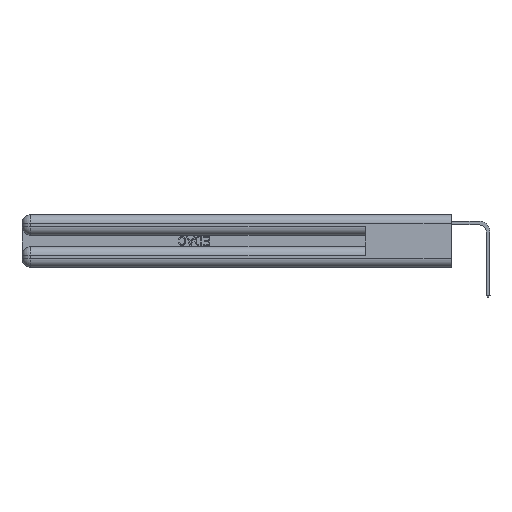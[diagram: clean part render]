
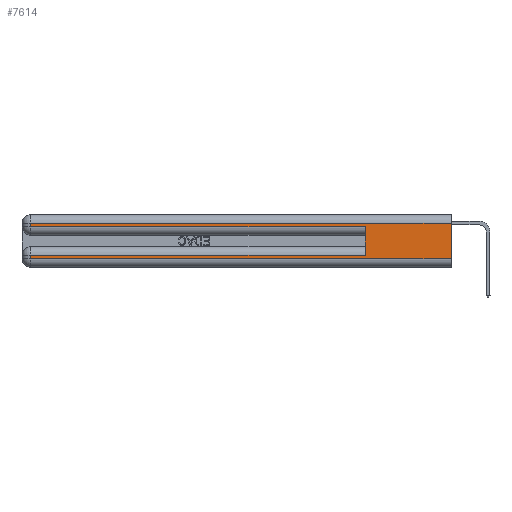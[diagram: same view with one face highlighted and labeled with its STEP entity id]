
A CAD part, left-side view. The second image highlights one B-rep face of the part: STEP entity #7614.
In plain terms, the highlighted planar face has unit normal (-1, 0, 0).
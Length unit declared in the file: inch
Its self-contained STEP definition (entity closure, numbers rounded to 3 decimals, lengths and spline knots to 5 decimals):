
#253 = CARTESIAN_POINT ( 'NONE',  ( 0., 2.94, 0.31 ) ) ;
#452 = VERTEX_POINT ( 'NONE', #21533 ) ;
#843 = EDGE_CURVE ( 'NONE', #30634, #452, #5601, .T. ) ;
#1030 = VERTEX_POINT ( 'NONE', #19496 ) ;
#1300 = EDGE_CURVE ( 'NONE', #452, #10364, #24338, .T. ) ;
#1355 = VECTOR ( 'NONE', #16055, 39.37008 ) ;
#1785 = VECTOR ( 'NONE', #31745, 39.37008 ) ;
#2226 = LINE ( 'NONE', #19199, #3964 ) ;
#2249 = CARTESIAN_POINT ( 'NONE',  ( 0., 0.6, 0.085 ) ) ;
#2489 = CARTESIAN_POINT ( 'NONE',  ( 0., 2.94, 0.37 ) ) ;
#3964 = VECTOR ( 'NONE', #19020, 39.37008 ) ;
#4305 = LINE ( 'NONE', #32068, #22374 ) ;
#4582 = EDGE_CURVE ( 'NONE', #30634, #18506, #25708, .T. ) ;
#4866 = CARTESIAN_POINT ( 'NONE',  ( 0., 2.94, 0.06 ) ) ;
#5601 = LINE ( 'NONE', #30299, #11284 ) ;
#5830 = VERTEX_POINT ( 'NONE', #34524 ) ;
#5873 = VECTOR ( 'NONE', #19997, 39.37008 ) ;
#7510 = VECTOR ( 'NONE', #20439, 39.37008 ) ;
#7595 = EDGE_CURVE ( 'NONE', #5830, #18506, #19461, .T. ) ;
#7614 = ADVANCED_FACE ( 'NONE', ( #24515 ), #13869, .F. ) ;
#9401 = EDGE_LOOP ( 'NONE', ( #22120, #16049, #32577, #11719, #10735, #12532, #11450, #30778 ) ) ;
#9784 = VERTEX_POINT ( 'NONE', #253 ) ;
#10364 = VERTEX_POINT ( 'NONE', #4866 ) ;
#10721 = VERTEX_POINT ( 'NONE', #23597 ) ;
#10735 = ORIENTED_EDGE ( 'NONE', *, *, #4582, .F. ) ;
#11284 = VECTOR ( 'NONE', #32482, 39.37008 ) ;
#11450 = ORIENTED_EDGE ( 'NONE', *, *, #1300, .T. ) ;
#11719 = ORIENTED_EDGE ( 'NONE', *, *, #7595, .T. ) ;
#12475 = VECTOR ( 'NONE', #23980, 39.37008 ) ;
#12532 = ORIENTED_EDGE ( 'NONE', *, *, #843, .T. ) ;
#13869 = PLANE ( 'NONE',  #31309 ) ;
#14878 = DIRECTION ( 'NONE',  ( 1., 0., 0. ) ) ;
#15865 = DIRECTION ( 'NONE',  ( 0., 1., 0. ) ) ;
#16049 = ORIENTED_EDGE ( 'NONE', *, *, #19455, .T. ) ;
#16055 = DIRECTION ( 'NONE',  ( 0., -1., 0. ) ) ;
#18438 = CARTESIAN_POINT ( 'NONE',  ( 0., 0., 0.37 ) ) ;
#18506 = VERTEX_POINT ( 'NONE', #25930 ) ;
#18752 = CARTESIAN_POINT ( 'NONE',  ( 0., 0., 0.285 ) ) ;
#19020 = DIRECTION ( 'NONE',  ( 0., 0., -1. ) ) ;
#19199 = CARTESIAN_POINT ( 'NONE',  ( 0., 2.94, 0.37 ) ) ;
#19455 = EDGE_CURVE ( 'NONE', #1030, #9784, #4305, .T. ) ;
#19461 = LINE ( 'NONE', #18752, #1355 ) ;
#19496 = CARTESIAN_POINT ( 'NONE',  ( 0., 0., 0.31 ) ) ;
#19997 = DIRECTION ( 'NONE',  ( 0., -1., 0. ) ) ;
#20356 = LINE ( 'NONE', #28660, #5873 ) ;
#20439 = DIRECTION ( 'NONE',  ( 0., 0., 1. ) ) ;
#20486 = EDGE_CURVE ( 'NONE', #9784, #5830, #2226, .T. ) ;
#21533 = CARTESIAN_POINT ( 'NONE',  ( 0., 2.94, 0.085 ) ) ;
#22120 = ORIENTED_EDGE ( 'NONE', *, *, #28405, .F. ) ;
#22374 = VECTOR ( 'NONE', #15865, 39.37008 ) ;
#23513 = CARTESIAN_POINT ( 'NONE',  ( 0., 0.6, 0.145 ) ) ;
#23597 = CARTESIAN_POINT ( 'NONE',  ( 0., 0., 0.06 ) ) ;
#23980 = DIRECTION ( 'NONE',  ( 0., 0., -1. ) ) ;
#24338 = LINE ( 'NONE', #2489, #12475 ) ;
#24515 = FACE_OUTER_BOUND ( 'NONE', #9401, .T. ) ;
#25708 = LINE ( 'NONE', #23513, #7510 ) ;
#25930 = CARTESIAN_POINT ( 'NONE',  ( 0., 0.6, 0.285 ) ) ;
#26569 = LINE ( 'NONE', #18438, #1785 ) ;
#28405 = EDGE_CURVE ( 'NONE', #1030, #10721, #26569, .T. ) ;
#28660 = CARTESIAN_POINT ( 'NONE',  ( 0., 0., 0.06 ) ) ;
#29739 = DIRECTION ( 'NONE',  ( 0., 0., -1. ) ) ;
#30299 = CARTESIAN_POINT ( 'NONE',  ( 0., 0., 0.085 ) ) ;
#30634 = VERTEX_POINT ( 'NONE', #2249 ) ;
#30778 = ORIENTED_EDGE ( 'NONE', *, *, #31165, .T. ) ;
#31165 = EDGE_CURVE ( 'NONE', #10364, #10721, #20356, .T. ) ;
#31309 = AXIS2_PLACEMENT_3D ( 'NONE', #35517, #14878, #29739 ) ;
#31745 = DIRECTION ( 'NONE',  ( 0., 0., -1. ) ) ;
#32068 = CARTESIAN_POINT ( 'NONE',  ( 0., 0., 0.31 ) ) ;
#32482 = DIRECTION ( 'NONE',  ( 0., 1., 0. ) ) ;
#32577 = ORIENTED_EDGE ( 'NONE', *, *, #20486, .T. ) ;
#34524 = CARTESIAN_POINT ( 'NONE',  ( 0., 2.94, 0.285 ) ) ;
#35517 = CARTESIAN_POINT ( 'NONE',  ( 0., 0., 0.37 ) ) ;
